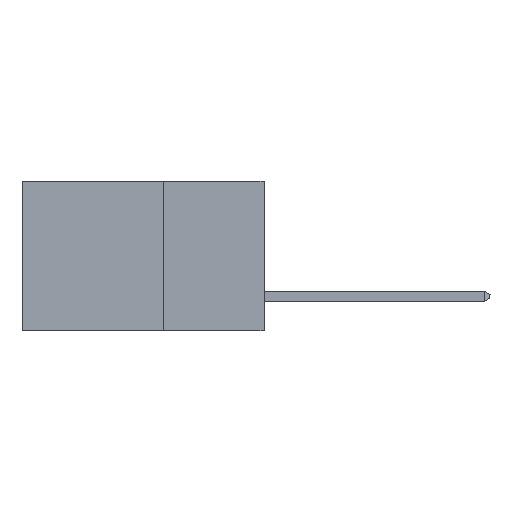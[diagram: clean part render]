
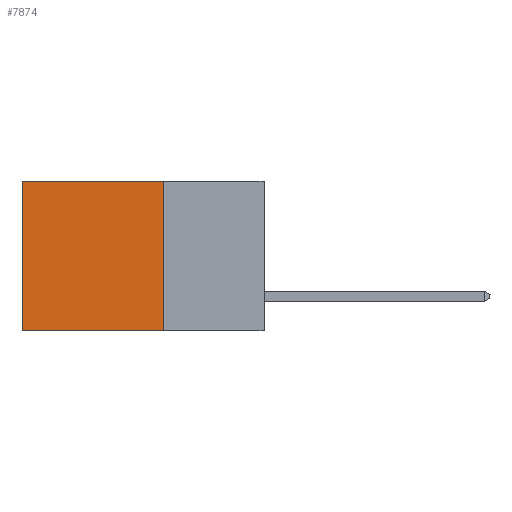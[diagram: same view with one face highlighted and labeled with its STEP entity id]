
A CAD part, left-side view. The second image highlights one B-rep face of the part: STEP entity #7874.
In plain terms, the highlighted planar face has unit normal (-1, 0, 0).
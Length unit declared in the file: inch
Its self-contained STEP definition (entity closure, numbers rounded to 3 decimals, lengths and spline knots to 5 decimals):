
#718 = LINE ( 'NONE', #810, #15547 ) ;
#810 = CARTESIAN_POINT ( 'NONE',  ( 0.2615, 0.25, -0.37 ) ) ;
#1113 = CARTESIAN_POINT ( 'NONE',  ( 0.2615, 0.25, -0.37 ) ) ;
#1130 = DIRECTION ( 'NONE',  ( 0., 1., 0. ) ) ;
#1509 = DIRECTION ( 'NONE',  ( 0., 0., -1. ) ) ;
#1718 = DIRECTION ( 'NONE',  ( 0., 1., 0. ) ) ;
#3609 = VERTEX_POINT ( 'NONE', #6121 ) ;
#4207 = CARTESIAN_POINT ( 'NONE',  ( 0.2615, 0.6, -0.37 ) ) ;
#4407 = EDGE_CURVE ( 'NONE', #15303, #9735, #15278, .T. ) ;
#4663 = VERTEX_POINT ( 'NONE', #9056 ) ;
#5535 = CARTESIAN_POINT ( 'NONE',  ( 0.2615, 0.25, 0. ) ) ;
#6029 = LINE ( 'NONE', #15305, #17285 ) ;
#6121 = CARTESIAN_POINT ( 'NONE',  ( 0.2615, 0.25, -0.37 ) ) ;
#6132 = ORIENTED_EDGE ( 'NONE', *, *, #14265, .T. ) ;
#6516 = DIRECTION ( 'NONE',  ( 0., 0., -1. ) ) ;
#6845 = EDGE_CURVE ( 'NONE', #4663, #3609, #718, .T. ) ;
#6879 = DIRECTION ( 'NONE',  ( 1., 0., 0. ) ) ;
#7874 = ADVANCED_FACE ( 'NONE', ( #17723 ), #17459, .F. ) ;
#7980 = LINE ( 'NONE', #5535, #17040 ) ;
#8570 = ORIENTED_EDGE ( 'NONE', *, *, #11157, .F. ) ;
#9056 = CARTESIAN_POINT ( 'NONE',  ( 0.2615, 0.25, 0. ) ) ;
#9735 = VERTEX_POINT ( 'NONE', #11250 ) ;
#10237 = DIRECTION ( 'NONE',  ( 0., 0., -1. ) ) ;
#10593 = VECTOR ( 'NONE', #1509, 39.37008 ) ;
#11072 = EDGE_LOOP ( 'NONE', ( #11985, #8570, #15557, #6132 ) ) ;
#11157 = EDGE_CURVE ( 'NONE', #3609, #9735, #6029, .T. ) ;
#11250 = CARTESIAN_POINT ( 'NONE',  ( 0.2615, 0.6, -0.37 ) ) ;
#11985 = ORIENTED_EDGE ( 'NONE', *, *, #4407, .T. ) ;
#13329 = AXIS2_PLACEMENT_3D ( 'NONE', #1113, #6879, #6516 ) ;
#14265 = EDGE_CURVE ( 'NONE', #4663, #15303, #7980, .T. ) ;
#14622 = CARTESIAN_POINT ( 'NONE',  ( 0.2615, 0.6, 0. ) ) ;
#15278 = LINE ( 'NONE', #4207, #10593 ) ;
#15303 = VERTEX_POINT ( 'NONE', #14622 ) ;
#15305 = CARTESIAN_POINT ( 'NONE',  ( 0.2615, 0.25, -0.37 ) ) ;
#15547 = VECTOR ( 'NONE', #10237, 39.37008 ) ;
#15557 = ORIENTED_EDGE ( 'NONE', *, *, #6845, .F. ) ;
#17040 = VECTOR ( 'NONE', #1130, 39.37008 ) ;
#17285 = VECTOR ( 'NONE', #1718, 39.37008 ) ;
#17459 = PLANE ( 'NONE',  #13329 ) ;
#17723 = FACE_OUTER_BOUND ( 'NONE', #11072, .T. ) ;
